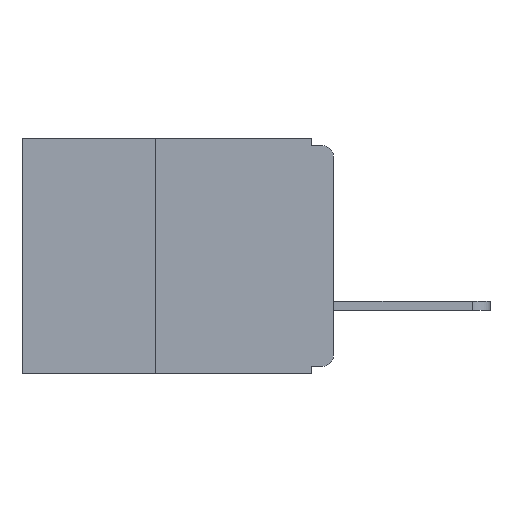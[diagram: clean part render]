
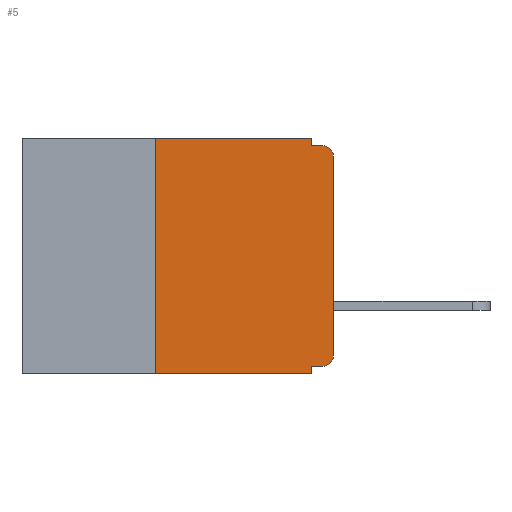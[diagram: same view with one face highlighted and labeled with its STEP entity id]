
A CAD part, left-side view. The second image highlights one B-rep face of the part: STEP entity #5.
In plain terms, the highlighted planar face has unit normal (-1, 0, 0).
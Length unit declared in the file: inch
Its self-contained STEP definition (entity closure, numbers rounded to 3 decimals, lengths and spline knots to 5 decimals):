
#5 = ADVANCED_FACE ( 'NONE', ( #8148 ), #6374, .F. ) ;
#63 = CARTESIAN_POINT ( 'NONE',  ( 0., 0.015, -0.025 ) ) ;
#113 = VERTEX_POINT ( 'NONE', #9374 ) ;
#373 = CARTESIAN_POINT ( 'NONE',  ( 0., 0., -0.01 ) ) ;
#435 = VERTEX_POINT ( 'NONE', #5224 ) ;
#644 = CARTESIAN_POINT ( 'NONE',  ( 0., 0.031, -0.33 ) ) ;
#875 = VECTOR ( 'NONE', #2875, 39.37008 ) ;
#1360 = EDGE_CURVE ( 'NONE', #8226, #11527, #2269, .T. ) ;
#1615 = VECTOR ( 'NONE', #3423, 39.37008 ) ;
#1706 = VERTEX_POINT ( 'NONE', #5246 ) ;
#1744 = DIRECTION ( 'NONE',  ( 1., 0., 0. ) ) ;
#1875 = DIRECTION ( 'NONE',  ( 0., 1., 0. ) ) ;
#1931 = DIRECTION ( 'NONE',  ( 0., 0., -1. ) ) ;
#2209 = LINE ( 'NONE', #9826, #1615 ) ;
#2269 = LINE ( 'NONE', #4302, #5513 ) ;
#2279 = EDGE_LOOP ( 'NONE', ( #5687, #5050, #7339, #9031, #7380, #3391, #11255, #10206, #6800, #8691 ) ) ;
#2755 = CARTESIAN_POINT ( 'NONE',  ( 0., 0.015, -0.305 ) ) ;
#2859 = CARTESIAN_POINT ( 'NONE',  ( 0., 0., -0.32 ) ) ;
#2875 = DIRECTION ( 'NONE',  ( 0., 0., -1. ) ) ;
#2929 = CIRCLE ( 'NONE', #6626, 0.015 ) ;
#2944 = EDGE_CURVE ( 'NONE', #113, #5952, #4307, .T. ) ;
#2963 = DIRECTION ( 'NONE',  ( 0., 0., 1. ) ) ;
#3130 = CARTESIAN_POINT ( 'NONE',  ( 0., 0., -0.025 ) ) ;
#3391 = ORIENTED_EDGE ( 'NONE', *, *, #11606, .F. ) ;
#3408 = VECTOR ( 'NONE', #7842, 39.37008 ) ;
#3423 = DIRECTION ( 'NONE',  ( 0., 0., 1. ) ) ;
#3780 = DIRECTION ( 'NONE',  ( -1., 0., 0. ) ) ;
#3829 = CARTESIAN_POINT ( 'NONE',  ( 0., 0.015, -0.32 ) ) ;
#3874 = VECTOR ( 'NONE', #9083, 39.37008 ) ;
#4073 = EDGE_CURVE ( 'NONE', #4690, #10280, #5453, .T. ) ;
#4106 = DIRECTION ( 'NONE',  ( 0., -1., 0. ) ) ;
#4302 = CARTESIAN_POINT ( 'NONE',  ( 0., 0.437, -0.33 ) ) ;
#4307 = LINE ( 'NONE', #10246, #9229 ) ;
#4690 = VERTEX_POINT ( 'NONE', #3829 ) ;
#5050 = ORIENTED_EDGE ( 'NONE', *, *, #10498, .T. ) ;
#5198 = EDGE_CURVE ( 'NONE', #4690, #113, #2929, .T. ) ;
#5224 = CARTESIAN_POINT ( 'NONE',  ( 0., 0.031, -0.01 ) ) ;
#5239 = CARTESIAN_POINT ( 'NONE',  ( 0., 0.031, -0.33 ) ) ;
#5246 = CARTESIAN_POINT ( 'NONE',  ( 0., 0.015, -0.01 ) ) ;
#5310 = EDGE_CURVE ( 'NONE', #9283, #435, #11325, .T. ) ;
#5453 = LINE ( 'NONE', #2859, #7912 ) ;
#5513 = VECTOR ( 'NONE', #7103, 39.37008 ) ;
#5687 = ORIENTED_EDGE ( 'NONE', *, *, #2944, .T. ) ;
#5894 = LINE ( 'NONE', #11384, #3408 ) ;
#5952 = VERTEX_POINT ( 'NONE', #3130 ) ;
#6119 = EDGE_CURVE ( 'NONE', #435, #1706, #9888, .T. ) ;
#6374 = PLANE ( 'NONE',  #10844 ) ;
#6411 = VECTOR ( 'NONE', #4106, 39.37008 ) ;
#6626 = AXIS2_PLACEMENT_3D ( 'NONE', #2755, #7415, #8002 ) ;
#6800 = ORIENTED_EDGE ( 'NONE', *, *, #4073, .F. ) ;
#7103 = DIRECTION ( 'NONE',  ( 0., -1., 0. ) ) ;
#7231 = CARTESIAN_POINT ( 'NONE',  ( 0., 0.25, -0.33 ) ) ;
#7339 = ORIENTED_EDGE ( 'NONE', *, *, #6119, .F. ) ;
#7380 = ORIENTED_EDGE ( 'NONE', *, *, #10106, .F. ) ;
#7415 = DIRECTION ( 'NONE',  ( -1., 0., 0. ) ) ;
#7842 = DIRECTION ( 'NONE',  ( 0., -1., 0. ) ) ;
#7912 = VECTOR ( 'NONE', #1875, 39.37008 ) ;
#8002 = DIRECTION ( 'NONE',  ( 0., 0., -1. ) ) ;
#8148 = FACE_OUTER_BOUND ( 'NONE', #2279, .T. ) ;
#8226 = VERTEX_POINT ( 'NONE', #7231 ) ;
#8257 = DIRECTION ( 'NONE',  ( 0., 0., -1. ) ) ;
#8405 = CARTESIAN_POINT ( 'NONE',  ( 0., 0.25, 0. ) ) ;
#8514 = LINE ( 'NONE', #5239, #3874 ) ;
#8691 = ORIENTED_EDGE ( 'NONE', *, *, #5198, .T. ) ;
#8817 = CARTESIAN_POINT ( 'NONE',  ( 0., 0.031, -0.32 ) ) ;
#8889 = AXIS2_PLACEMENT_3D ( 'NONE', #63, #3780, #1931 ) ;
#9031 = ORIENTED_EDGE ( 'NONE', *, *, #5310, .F. ) ;
#9083 = DIRECTION ( 'NONE',  ( 0., 0., -1. ) ) ;
#9229 = VECTOR ( 'NONE', #2963, 39.37008 ) ;
#9232 = EDGE_CURVE ( 'NONE', #10280, #11527, #8514, .T. ) ;
#9283 = VERTEX_POINT ( 'NONE', #9986 ) ;
#9374 = CARTESIAN_POINT ( 'NONE',  ( 0., 0., -0.305 ) ) ;
#9826 = CARTESIAN_POINT ( 'NONE',  ( 0., 0.25, -0.33 ) ) ;
#9888 = LINE ( 'NONE', #373, #6411 ) ;
#9986 = CARTESIAN_POINT ( 'NONE',  ( 0., 0.031, 0. ) ) ;
#10106 = EDGE_CURVE ( 'NONE', #10495, #9283, #5894, .T. ) ;
#10172 = CARTESIAN_POINT ( 'NONE',  ( 0., 0.437, 0. ) ) ;
#10190 = CIRCLE ( 'NONE', #8889, 0.015 ) ;
#10206 = ORIENTED_EDGE ( 'NONE', *, *, #9232, .F. ) ;
#10246 = CARTESIAN_POINT ( 'NONE',  ( 0., 0., 0. ) ) ;
#10280 = VERTEX_POINT ( 'NONE', #8817 ) ;
#10495 = VERTEX_POINT ( 'NONE', #8405 ) ;
#10498 = EDGE_CURVE ( 'NONE', #5952, #1706, #10190, .T. ) ;
#10844 = AXIS2_PLACEMENT_3D ( 'NONE', #10172, #1744, #8257 ) ;
#11255 = ORIENTED_EDGE ( 'NONE', *, *, #1360, .T. ) ;
#11285 = CARTESIAN_POINT ( 'NONE',  ( 0., 0.031, 0. ) ) ;
#11325 = LINE ( 'NONE', #11285, #875 ) ;
#11384 = CARTESIAN_POINT ( 'NONE',  ( 0., 0.437, 0. ) ) ;
#11527 = VERTEX_POINT ( 'NONE', #644 ) ;
#11606 = EDGE_CURVE ( 'NONE', #8226, #10495, #2209, .T. ) ;
